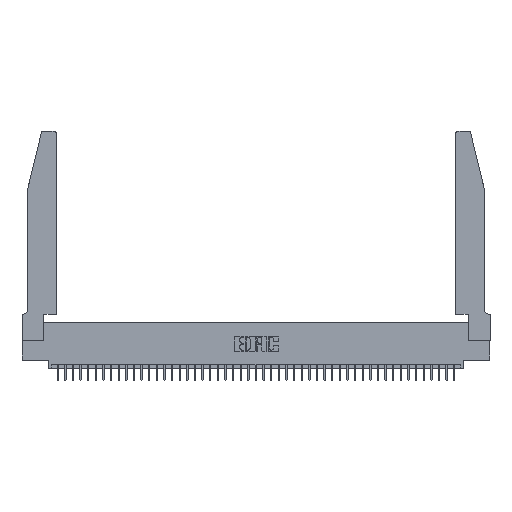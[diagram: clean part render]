
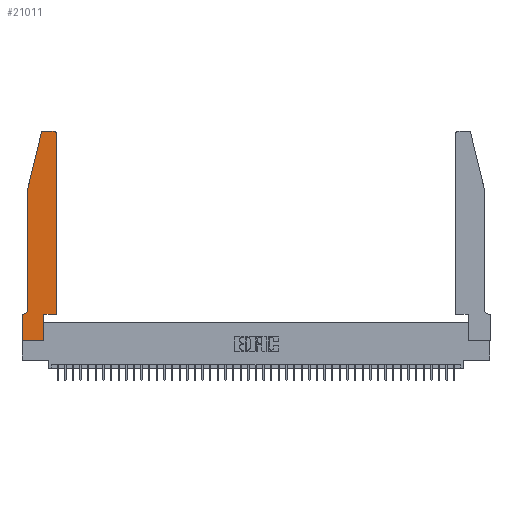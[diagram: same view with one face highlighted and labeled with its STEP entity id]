
A CAD part, top view. The second image highlights one B-rep face of the part: STEP entity #21011.
In plain terms, the highlighted planar face has unit normal (0, 0, 1).
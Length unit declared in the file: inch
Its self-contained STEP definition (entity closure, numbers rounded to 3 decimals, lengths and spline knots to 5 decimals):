
#194 = VERTEX_POINT ( 'NONE', #34912 ) ;
#803 = DIRECTION ( 'NONE',  ( 1., 0., 0. ) ) ;
#954 = LINE ( 'NONE', #27873, #36996 ) ;
#2101 = EDGE_CURVE ( 'NONE', #31456, #35568, #30013, .T. ) ;
#2254 = CARTESIAN_POINT ( 'NONE',  ( 0.2865, 0.35, 0.37 ) ) ;
#2307 = CARTESIAN_POINT ( 'NONE',  ( 0., 0., 0.37 ) ) ;
#3408 = CARTESIAN_POINT ( 'NONE',  ( 0., 0.35, 0.37 ) ) ;
#3533 = VERTEX_POINT ( 'NONE', #42957 ) ;
#4155 = DIRECTION ( 'NONE',  ( 1., 0., 0. ) ) ;
#4273 = EDGE_CURVE ( 'NONE', #40779, #29425, #38018, .T. ) ;
#4752 = DIRECTION ( 'NONE',  ( 0., -1., 0. ) ) ;
#5112 = CARTESIAN_POINT ( 'NONE',  ( 0.284, 2.72, 0.37 ) ) ;
#5153 = AXIS2_PLACEMENT_3D ( 'NONE', #9852, #21202, #24261 ) ;
#5423 = DIRECTION ( 'NONE',  ( 1., 0., 0. ) ) ;
#6199 = ORIENTED_EDGE ( 'NONE', *, *, #43976, .T. ) ;
#6422 = ORIENTED_EDGE ( 'NONE', *, *, #30399, .T. ) ;
#7595 = CARTESIAN_POINT ( 'NONE',  ( 0.0755, 2., 0.37 ) ) ;
#7735 = VERTEX_POINT ( 'NONE', #3408 ) ;
#8276 = EDGE_CURVE ( 'NONE', #7735, #29402, #44855, .T. ) ;
#8549 = VECTOR ( 'NONE', #26629, 39.37008 ) ;
#8873 = VERTEX_POINT ( 'NONE', #19427 ) ;
#9051 = CARTESIAN_POINT ( 'NONE',  ( 0.25487, 2.72718, 0.37 ) ) ;
#9267 = LINE ( 'NONE', #41191, #23941 ) ;
#9852 = CARTESIAN_POINT ( 'NONE',  ( 0.0055, 0.42, 0.37 ) ) ;
#9960 = EDGE_CURVE ( 'NONE', #35568, #3533, #22268, .T. ) ;
#11454 = CARTESIAN_POINT ( 'NONE',  ( 0., 0., 0.37 ) ) ;
#12277 = DIRECTION ( 'NONE',  ( 0., 0., 1. ) ) ;
#12776 = ORIENTED_EDGE ( 'NONE', *, *, #4273, .T. ) ;
#12805 = DIRECTION ( 'NONE',  ( -0.239, -0.971, 0. ) ) ;
#13437 = CARTESIAN_POINT ( 'NONE',  ( 0.0755, 2., 0.37 ) ) ;
#16176 = ORIENTED_EDGE ( 'NONE', *, *, #17304, .T. ) ;
#16755 = FACE_OUTER_BOUND ( 'NONE', #31807, .T. ) ;
#17262 = VECTOR ( 'NONE', #12805, 39.37008 ) ;
#17304 = EDGE_CURVE ( 'NONE', #28760, #31456, #29447, .T. ) ;
#17419 = CIRCLE ( 'NONE', #24833, 0.03 ) ;
#17468 = EDGE_CURVE ( 'NONE', #29425, #8873, #9267, .T. ) ;
#17832 = PLANE ( 'NONE',  #19681 ) ;
#17915 = ORIENTED_EDGE ( 'NONE', *, *, #9960, .T. ) ;
#19075 = CARTESIAN_POINT ( 'NONE',  ( 0.4205, 2.72, 0.37 ) ) ;
#19164 = CARTESIAN_POINT ( 'NONE',  ( 0.2605, 2.75, 0.37 ) ) ;
#19179 = ORIENTED_EDGE ( 'NONE', *, *, #23108, .T. ) ;
#19427 = CARTESIAN_POINT ( 'NONE',  ( 0.0755, 0.42, 0.37 ) ) ;
#19431 = DIRECTION ( 'NONE',  ( 0., 1., 0. ) ) ;
#19531 = CARTESIAN_POINT ( 'NONE',  ( 0.4505, 0.35, 0.37 ) ) ;
#19681 = AXIS2_PLACEMENT_3D ( 'NONE', #21473, #25292, #4155 ) ;
#20669 = ORIENTED_EDGE ( 'NONE', *, *, #17468, .T. ) ;
#21011 = ADVANCED_FACE ( 'NONE', ( #16755 ), #17832, .T. ) ;
#21178 = VECTOR ( 'NONE', #26638, 39.37008 ) ;
#21202 = DIRECTION ( 'NONE',  ( 0., 0., -1. ) ) ;
#21473 = CARTESIAN_POINT ( 'NONE',  ( 0., 0.35, 0.37 ) ) ;
#21796 = CARTESIAN_POINT ( 'NONE',  ( 0.4505, 0.35, 0.37 ) ) ;
#22268 = LINE ( 'NONE', #19164, #21178 ) ;
#23062 = CIRCLE ( 'NONE', #5153, 0.07 ) ;
#23108 = EDGE_CURVE ( 'NONE', #8873, #194, #23062, .T. ) ;
#23941 = VECTOR ( 'NONE', #24045, 39.37008 ) ;
#24037 = DIRECTION ( 'NONE',  ( -1., 0., 0. ) ) ;
#24045 = DIRECTION ( 'NONE',  ( 0., -1., 0. ) ) ;
#24261 = DIRECTION ( 'NONE',  ( -1., 0., 0. ) ) ;
#24833 = AXIS2_PLACEMENT_3D ( 'NONE', #5112, #26421, #5423 ) ;
#25292 = DIRECTION ( 'NONE',  ( 0., 0., 1. ) ) ;
#25298 = AXIS2_PLACEMENT_3D ( 'NONE', #19075, #12277, #36641 ) ;
#26421 = DIRECTION ( 'NONE',  ( 0., 0., 1. ) ) ;
#26629 = DIRECTION ( 'NONE',  ( 1., 0., 0. ) ) ;
#26638 = DIRECTION ( 'NONE',  ( -1., 0., 0. ) ) ;
#26897 = CARTESIAN_POINT ( 'NONE',  ( 0.2865, 0.35, 0.37 ) ) ;
#27002 = ORIENTED_EDGE ( 'NONE', *, *, #30560, .T. ) ;
#27774 = VECTOR ( 'NONE', #44243, 39.37008 ) ;
#27873 = CARTESIAN_POINT ( 'NONE',  ( 0.0755, 0.35, 0.37 ) ) ;
#28760 = VERTEX_POINT ( 'NONE', #30245 ) ;
#29247 = LINE ( 'NONE', #2307, #8549 ) ;
#29402 = VERTEX_POINT ( 'NONE', #44382 ) ;
#29425 = VERTEX_POINT ( 'NONE', #13437 ) ;
#29447 = LINE ( 'NONE', #19531, #27774 ) ;
#29689 = LINE ( 'NONE', #26897, #30751 ) ;
#30013 = CIRCLE ( 'NONE', #25298, 0.03 ) ;
#30245 = CARTESIAN_POINT ( 'NONE',  ( 0.4505, 0.35, 0.37 ) ) ;
#30399 = EDGE_CURVE ( 'NONE', #41901, #28760, #42543, .T. ) ;
#30414 = CARTESIAN_POINT ( 'NONE',  ( 0.4205, 2.75, 0.37 ) ) ;
#30550 = CARTESIAN_POINT ( 'NONE',  ( 0.2865, 0., 0.37 ) ) ;
#30560 = EDGE_CURVE ( 'NONE', #3533, #40779, #17419, .T. ) ;
#30751 = VECTOR ( 'NONE', #19431, 39.37008 ) ;
#31456 = VERTEX_POINT ( 'NONE', #38032 ) ;
#31807 = EDGE_LOOP ( 'NONE', ( #17915, #27002, #12776, #20669, #19179, #36427, #36703, #6199, #34739, #6422, #16176, #32662 ) ) ;
#32662 = ORIENTED_EDGE ( 'NONE', *, *, #2101, .T. ) ;
#33398 = VECTOR ( 'NONE', #4752, 39.37008 ) ;
#34559 = EDGE_CURVE ( 'NONE', #194, #7735, #954, .T. ) ;
#34739 = ORIENTED_EDGE ( 'NONE', *, *, #36973, .T. ) ;
#34912 = CARTESIAN_POINT ( 'NONE',  ( 0.0055, 0.35, 0.37 ) ) ;
#35568 = VERTEX_POINT ( 'NONE', #30414 ) ;
#36427 = ORIENTED_EDGE ( 'NONE', *, *, #34559, .T. ) ;
#36641 = DIRECTION ( 'NONE',  ( 1., 0., 0. ) ) ;
#36703 = ORIENTED_EDGE ( 'NONE', *, *, #8276, .T. ) ;
#36973 = EDGE_CURVE ( 'NONE', #37145, #41901, #29689, .T. ) ;
#36996 = VECTOR ( 'NONE', #24037, 39.37008 ) ;
#37145 = VERTEX_POINT ( 'NONE', #30550 ) ;
#38018 = LINE ( 'NONE', #7595, #17262 ) ;
#38032 = CARTESIAN_POINT ( 'NONE',  ( 0.4505, 2.72, 0.37 ) ) ;
#40779 = VERTEX_POINT ( 'NONE', #9051 ) ;
#40911 = VECTOR ( 'NONE', #803, 39.37008 ) ;
#41191 = CARTESIAN_POINT ( 'NONE',  ( 0.0755, 2., 0.37 ) ) ;
#41901 = VERTEX_POINT ( 'NONE', #2254 ) ;
#42543 = LINE ( 'NONE', #21796, #40911 ) ;
#42957 = CARTESIAN_POINT ( 'NONE',  ( 0.284, 2.75, 0.37 ) ) ;
#43976 = EDGE_CURVE ( 'NONE', #29402, #37145, #29247, .T. ) ;
#44243 = DIRECTION ( 'NONE',  ( 0., 1., 0. ) ) ;
#44382 = CARTESIAN_POINT ( 'NONE',  ( 0., 0., 0.37 ) ) ;
#44855 = LINE ( 'NONE', #11454, #33398 ) ;
